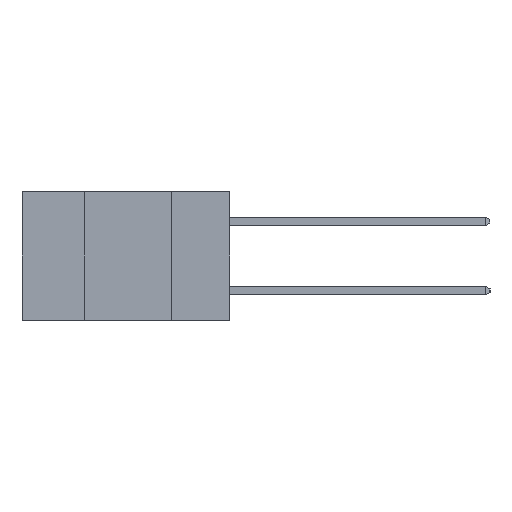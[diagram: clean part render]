
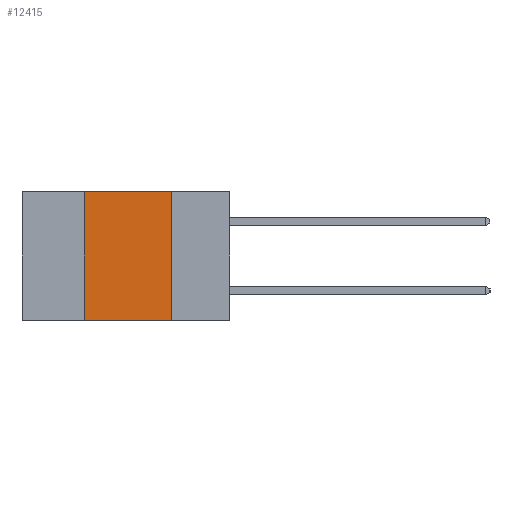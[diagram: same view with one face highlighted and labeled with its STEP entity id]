
A CAD part, left-side view. The second image highlights one B-rep face of the part: STEP entity #12415.
In plain terms, the highlighted planar face has unit normal (-1, 0, 0).
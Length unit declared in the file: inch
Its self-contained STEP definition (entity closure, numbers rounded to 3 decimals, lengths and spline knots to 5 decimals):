
#387 = DIRECTION ( 'NONE',  ( 1., 0., 0. ) ) ;
#433 = DIRECTION ( 'NONE',  ( 0., 0., -1. ) ) ;
#1647 = VECTOR ( 'NONE', #16642, 39.37008 ) ;
#2012 = CARTESIAN_POINT ( 'NONE',  ( 0., 0.42, 0. ) ) ;
#3716 = PLANE ( 'NONE',  #21639 ) ;
#4194 = VERTEX_POINT ( 'NONE', #14948 ) ;
#4299 = VECTOR ( 'NONE', #6259, 39.37008 ) ;
#4986 = CARTESIAN_POINT ( 'NONE',  ( 0., 0.6, -0.37 ) ) ;
#5006 = ORIENTED_EDGE ( 'NONE', *, *, #20374, .F. ) ;
#5032 = DIRECTION ( 'NONE',  ( 0., -1., 0. ) ) ;
#6259 = DIRECTION ( 'NONE',  ( 0., -1., 0. ) ) ;
#6471 = LINE ( 'NONE', #4986, #19565 ) ;
#6636 = CARTESIAN_POINT ( 'NONE',  ( 0., 0.42, -0.37 ) ) ;
#6760 = CARTESIAN_POINT ( 'NONE',  ( 0., 0.6, 0. ) ) ;
#6792 = EDGE_CURVE ( 'NONE', #14119, #20940, #6471, .T. ) ;
#7774 = EDGE_CURVE ( 'NONE', #10902, #4194, #8819, .T. ) ;
#7924 = EDGE_CURVE ( 'NONE', #14119, #10902, #15218, .T. ) ;
#8457 = ORIENTED_EDGE ( 'NONE', *, *, #6792, .T. ) ;
#8819 = LINE ( 'NONE', #6760, #4299 ) ;
#8979 = ORIENTED_EDGE ( 'NONE', *, *, #7924, .F. ) ;
#9121 = VECTOR ( 'NONE', #433, 39.37008 ) ;
#10537 = CARTESIAN_POINT ( 'NONE',  ( 0., 0.6, 0. ) ) ;
#10902 = VERTEX_POINT ( 'NONE', #2012 ) ;
#12243 = DIRECTION ( 'NONE',  ( 0., 0., -1. ) ) ;
#12415 = ADVANCED_FACE ( 'NONE', ( #16468 ), #3716, .F. ) ;
#13394 = CARTESIAN_POINT ( 'NONE',  ( 0., 0.17, -0.37 ) ) ;
#14119 = VERTEX_POINT ( 'NONE', #6636 ) ;
#14177 = LINE ( 'NONE', #19147, #9121 ) ;
#14948 = CARTESIAN_POINT ( 'NONE',  ( 0., 0.17, 0. ) ) ;
#15218 = LINE ( 'NONE', #15469, #1647 ) ;
#15469 = CARTESIAN_POINT ( 'NONE',  ( 0., 0.42, -0.37 ) ) ;
#15512 = EDGE_LOOP ( 'NONE', ( #5006, #18073, #8979, #8457 ) ) ;
#16468 = FACE_OUTER_BOUND ( 'NONE', #15512, .T. ) ;
#16642 = DIRECTION ( 'NONE',  ( 0., 0., 1. ) ) ;
#18073 = ORIENTED_EDGE ( 'NONE', *, *, #7774, .F. ) ;
#19147 = CARTESIAN_POINT ( 'NONE',  ( 0., 0.17, -0.37 ) ) ;
#19565 = VECTOR ( 'NONE', #5032, 39.37008 ) ;
#20374 = EDGE_CURVE ( 'NONE', #4194, #20940, #14177, .T. ) ;
#20940 = VERTEX_POINT ( 'NONE', #13394 ) ;
#21639 = AXIS2_PLACEMENT_3D ( 'NONE', #10537, #387, #12243 ) ;
